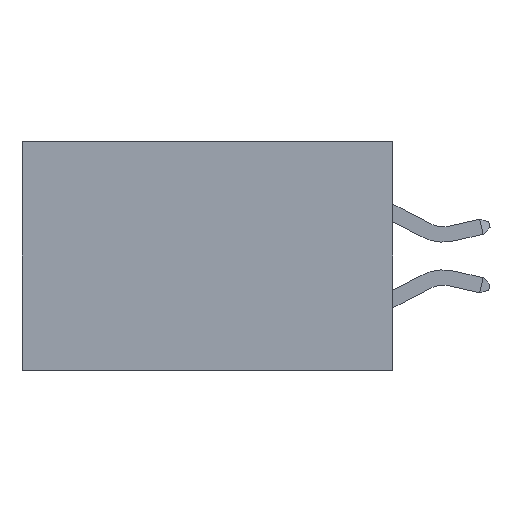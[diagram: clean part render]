
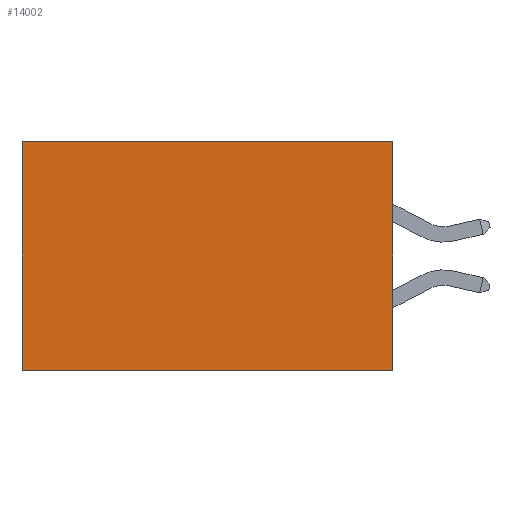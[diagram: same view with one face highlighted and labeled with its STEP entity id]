
A CAD part, left-side view. The second image highlights one B-rep face of the part: STEP entity #14002.
In plain terms, the highlighted planar face has unit normal (-1, 0, 0).
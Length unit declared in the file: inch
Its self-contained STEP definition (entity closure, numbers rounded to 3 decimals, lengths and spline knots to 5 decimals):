
#348 = EDGE_CURVE ( 'NONE', #24486, #25217, #12476, .T. ) ;
#449 = DIRECTION ( 'NONE',  ( 0., 1., 0. ) ) ;
#1559 = LINE ( 'NONE', #17059, #12224 ) ;
#1780 = PLANE ( 'NONE',  #29866 ) ;
#1946 = ORIENTED_EDGE ( 'NONE', *, *, #7634, .F. ) ;
#2227 = ORIENTED_EDGE ( 'NONE', *, *, #27272, .F. ) ;
#3300 = LINE ( 'NONE', #21550, #16142 ) ;
#4488 = EDGE_CURVE ( 'NONE', #7083, #24486, #3300, .T. ) ;
#7083 = VERTEX_POINT ( 'NONE', #12856 ) ;
#7494 = CARTESIAN_POINT ( 'NONE',  ( 0.2875, 0., 0. ) ) ;
#7634 = EDGE_CURVE ( 'NONE', #7083, #18774, #13374, .T. ) ;
#9180 = DIRECTION ( 'NONE',  ( 1., 0., 0. ) ) ;
#9299 = CARTESIAN_POINT ( 'NONE',  ( 0.2875, 0.6, 0. ) ) ;
#9567 = CARTESIAN_POINT ( 'NONE',  ( 0.2875, 0.6, -0.37 ) ) ;
#10520 = EDGE_LOOP ( 'NONE', ( #22038, #2227, #1946, #11878 ) ) ;
#11878 = ORIENTED_EDGE ( 'NONE', *, *, #4488, .T. ) ;
#12224 = VECTOR ( 'NONE', #28910, 39.37008 ) ;
#12476 = LINE ( 'NONE', #28827, #24287 ) ;
#12856 = CARTESIAN_POINT ( 'NONE',  ( 0.2875, 0., 0. ) ) ;
#13374 = LINE ( 'NONE', #7494, #18903 ) ;
#14002 = ADVANCED_FACE ( 'NONE', ( #18393 ), #1780, .F. ) ;
#16142 = VECTOR ( 'NONE', #449, 39.37008 ) ;
#17059 = CARTESIAN_POINT ( 'NONE',  ( 0.2875, 0., -0.37 ) ) ;
#18393 = FACE_OUTER_BOUND ( 'NONE', #10520, .T. ) ;
#18774 = VERTEX_POINT ( 'NONE', #28189 ) ;
#18903 = VECTOR ( 'NONE', #26440, 39.37008 ) ;
#21550 = CARTESIAN_POINT ( 'NONE',  ( 0.2875, 0., 0. ) ) ;
#22038 = ORIENTED_EDGE ( 'NONE', *, *, #348, .T. ) ;
#23387 = CARTESIAN_POINT ( 'NONE',  ( 0.2875, 0., 0. ) ) ;
#24073 = DIRECTION ( 'NONE',  ( 0., 0., -1. ) ) ;
#24287 = VECTOR ( 'NONE', #24073, 39.37008 ) ;
#24486 = VERTEX_POINT ( 'NONE', #9299 ) ;
#25217 = VERTEX_POINT ( 'NONE', #9567 ) ;
#25747 = DIRECTION ( 'NONE',  ( 0., 0., -1. ) ) ;
#26440 = DIRECTION ( 'NONE',  ( 0., 0., -1. ) ) ;
#27272 = EDGE_CURVE ( 'NONE', #18774, #25217, #1559, .T. ) ;
#28189 = CARTESIAN_POINT ( 'NONE',  ( 0.2875, 0., -0.37 ) ) ;
#28827 = CARTESIAN_POINT ( 'NONE',  ( 0.2875, 0.6, 0. ) ) ;
#28910 = DIRECTION ( 'NONE',  ( 0., 1., 0. ) ) ;
#29866 = AXIS2_PLACEMENT_3D ( 'NONE', #23387, #9180, #25747 ) ;
